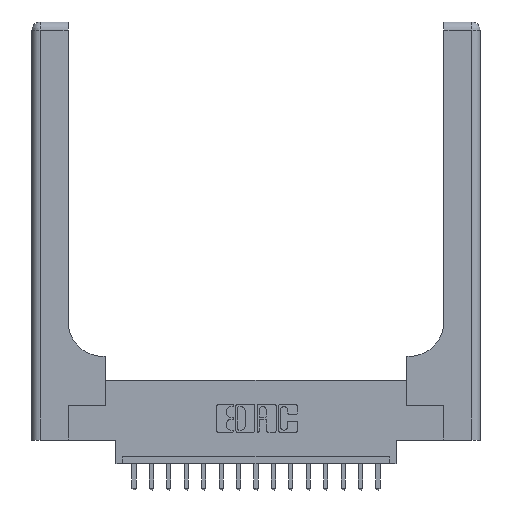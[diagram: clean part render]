
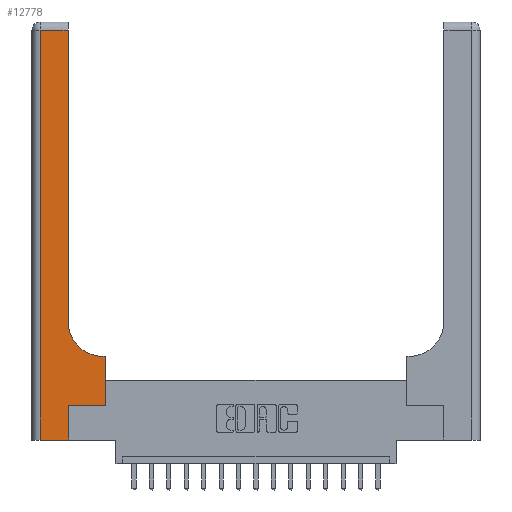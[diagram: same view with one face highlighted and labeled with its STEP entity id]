
A CAD part, top view. The second image highlights one B-rep face of the part: STEP entity #12778.
In plain terms, the highlighted planar face has unit normal (0, 0, 1).
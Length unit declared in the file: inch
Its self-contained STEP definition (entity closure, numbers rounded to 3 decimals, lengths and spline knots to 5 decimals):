
#297 = CARTESIAN_POINT ( 'NONE',  ( 0.528, 0.25, 0.37 ) ) ;
#462 = CARTESIAN_POINT ( 'NONE',  ( 0.265, 0.25, 0.37 ) ) ;
#751 = DIRECTION ( 'NONE',  ( 0., 1., 0. ) ) ;
#1120 = VECTOR ( 'NONE', #751, 39.37008 ) ;
#1301 = CARTESIAN_POINT ( 'NONE',  ( 0., 0., 0.37 ) ) ;
#1485 = EDGE_CURVE ( 'NONE', #12493, #12645, #3928, .T. ) ;
#1633 = CARTESIAN_POINT ( 'NONE',  ( 0.528, 0.25, 0.37 ) ) ;
#1840 = AXIS2_PLACEMENT_3D ( 'NONE', #9301, #18042, #2161 ) ;
#2161 = DIRECTION ( 'NONE',  ( -1., 0., 0. ) ) ;
#2319 = LINE ( 'NONE', #12432, #15719 ) ;
#2507 = CARTESIAN_POINT ( 'NONE',  ( 0.51, 0.6, 0.37 ) ) ;
#2616 = VECTOR ( 'NONE', #8704, 39.37008 ) ;
#3251 = LINE ( 'NONE', #297, #4597 ) ;
#3928 = LINE ( 'NONE', #14104, #4449 ) ;
#4239 = DIRECTION ( 'NONE',  ( 0., 0., -1. ) ) ;
#4449 = VECTOR ( 'NONE', #6961, 39.37008 ) ;
#4597 = VECTOR ( 'NONE', #4952, 39.37008 ) ;
#4952 = DIRECTION ( 'NONE',  ( 0., 1., 0. ) ) ;
#4957 = ORIENTED_EDGE ( 'NONE', *, *, #12934, .T. ) ;
#5130 = LINE ( 'NONE', #5514, #6273 ) ;
#5196 = ORIENTED_EDGE ( 'NONE', *, *, #16673, .T. ) ;
#5272 = DIRECTION ( 'NONE',  ( -1., 0., 0. ) ) ;
#5409 = VERTEX_POINT ( 'NONE', #1633 ) ;
#5514 = CARTESIAN_POINT ( 'NONE',  ( 0., 2.94, 0.37 ) ) ;
#6091 = AXIS2_PLACEMENT_3D ( 'NONE', #17261, #4239, #10039 ) ;
#6273 = VECTOR ( 'NONE', #11315, 39.37008 ) ;
#6686 = DIRECTION ( 'NONE',  ( 0., 1., 0. ) ) ;
#6929 = EDGE_CURVE ( 'NONE', #11201, #10679, #8094, .T. ) ;
#6961 = DIRECTION ( 'NONE',  ( 0., -1., 0. ) ) ;
#7066 = VERTEX_POINT ( 'NONE', #10387 ) ;
#7404 = DIRECTION ( 'NONE',  ( 1., 0., 0. ) ) ;
#7545 = EDGE_CURVE ( 'NONE', #7066, #5409, #7678, .T. ) ;
#7678 = LINE ( 'NONE', #462, #10551 ) ;
#7960 = LINE ( 'NONE', #13791, #1120 ) ;
#8032 = FACE_OUTER_BOUND ( 'NONE', #12350, .T. ) ;
#8094 = LINE ( 'NONE', #16856, #16313 ) ;
#8317 = ORIENTED_EDGE ( 'NONE', *, *, #17305, .T. ) ;
#8568 = ORIENTED_EDGE ( 'NONE', *, *, #7545, .T. ) ;
#8704 = DIRECTION ( 'NONE',  ( 1., 0., 0. ) ) ;
#9301 = CARTESIAN_POINT ( 'NONE',  ( 0., 3., 0.37 ) ) ;
#9506 = CARTESIAN_POINT ( 'NONE',  ( 0.06, 2.94, 0.37 ) ) ;
#10039 = DIRECTION ( 'NONE',  ( 1., 0., 0. ) ) ;
#10372 = VERTEX_POINT ( 'NONE', #2507 ) ;
#10387 = CARTESIAN_POINT ( 'NONE',  ( 0.265, 0.25, 0.37 ) ) ;
#10551 = VECTOR ( 'NONE', #7404, 39.37008 ) ;
#10679 = VERTEX_POINT ( 'NONE', #15502 ) ;
#11133 = ORIENTED_EDGE ( 'NONE', *, *, #13374, .T. ) ;
#11201 = VERTEX_POINT ( 'NONE', #12844 ) ;
#11315 = DIRECTION ( 'NONE',  ( -1., 0., 0. ) ) ;
#12184 = PLANE ( 'NONE',  #1840 ) ;
#12350 = EDGE_LOOP ( 'NONE', ( #15757, #8317, #12393, #5196, #18413, #8568, #11133, #12457, #4957 ) ) ;
#12393 = ORIENTED_EDGE ( 'NONE', *, *, #1485, .T. ) ;
#12432 = CARTESIAN_POINT ( 'NONE',  ( 0.26, 0.6, 0.37 ) ) ;
#12457 = ORIENTED_EDGE ( 'NONE', *, *, #18067, .T. ) ;
#12493 = VERTEX_POINT ( 'NONE', #9506 ) ;
#12635 = CARTESIAN_POINT ( 'NONE',  ( 0.528, 0.6, 0.37 ) ) ;
#12645 = VERTEX_POINT ( 'NONE', #13598 ) ;
#12778 = ADVANCED_FACE ( 'NONE', ( #8032 ), #12184, .F. ) ;
#12842 = VERTEX_POINT ( 'NONE', #13280 ) ;
#12844 = CARTESIAN_POINT ( 'NONE',  ( 0.26, 0.85, 0.37 ) ) ;
#12934 = EDGE_CURVE ( 'NONE', #10372, #11201, #14296, .T. ) ;
#13280 = CARTESIAN_POINT ( 'NONE',  ( 0.265, 0., 0.37 ) ) ;
#13374 = EDGE_CURVE ( 'NONE', #5409, #15615, #3251, .T. ) ;
#13598 = CARTESIAN_POINT ( 'NONE',  ( 0.06, 0., 0.37 ) ) ;
#13791 = CARTESIAN_POINT ( 'NONE',  ( 0.265, 0., 0.37 ) ) ;
#14104 = CARTESIAN_POINT ( 'NONE',  ( 0.06, 3., 0.37 ) ) ;
#14296 = CIRCLE ( 'NONE', #6091, 0.25 ) ;
#14331 = LINE ( 'NONE', #1301, #2616 ) ;
#15502 = CARTESIAN_POINT ( 'NONE',  ( 0.26, 2.94, 0.37 ) ) ;
#15615 = VERTEX_POINT ( 'NONE', #12635 ) ;
#15719 = VECTOR ( 'NONE', #5272, 39.37008 ) ;
#15757 = ORIENTED_EDGE ( 'NONE', *, *, #6929, .T. ) ;
#16313 = VECTOR ( 'NONE', #6686, 39.37008 ) ;
#16673 = EDGE_CURVE ( 'NONE', #12645, #12842, #14331, .T. ) ;
#16856 = CARTESIAN_POINT ( 'NONE',  ( 0.26, 3., 0.37 ) ) ;
#17261 = CARTESIAN_POINT ( 'NONE',  ( 0.51, 0.85, 0.37 ) ) ;
#17292 = EDGE_CURVE ( 'NONE', #12842, #7066, #7960, .T. ) ;
#17305 = EDGE_CURVE ( 'NONE', #10679, #12493, #5130, .T. ) ;
#18042 = DIRECTION ( 'NONE',  ( 0., 0., -1. ) ) ;
#18067 = EDGE_CURVE ( 'NONE', #15615, #10372, #2319, .T. ) ;
#18413 = ORIENTED_EDGE ( 'NONE', *, *, #17292, .T. ) ;
